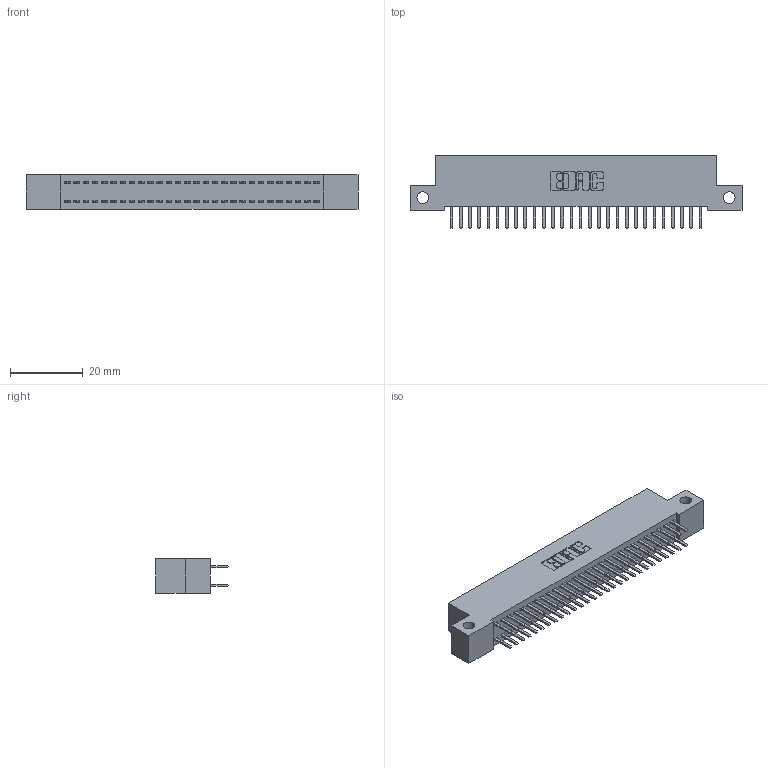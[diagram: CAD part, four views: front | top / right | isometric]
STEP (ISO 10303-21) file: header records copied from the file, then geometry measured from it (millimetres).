
FILE_DESCRIPTION (( 'STEP AP203' ), '1' );
FILE_NAME ('392-056-520-212.STEP', '2019-10-08T14:47:47', ( '' ), ( '' ), 'SwSTEP 2.0', 'SolidWorks 2016', '' );
FILE_SCHEMA (( 'CONFIG_CONTROL_DESIGN' ));
Length unit declared in the file: inch
Products named in the file (3): 342 Part_Side Mount; 345-292-001_345-293-120; 392-056-520-212
Assembly tree (57 placements, depth 2):
  392-056-520-212
    342 Part_Side Mount
    345-292-001_345-293-120  x56
Bounding box: 91.44 x 20.02 x 9.4 mm (x, y, z)
Volume: 8051.1 mm3; surface area: 12542.3 mm2
Topology: 57 solids, 57 shells, 3246 faces, 9427 edges, 6134 vertices
Faces by surface type: plane 2194, cylinder 1052
Entity records: 19809 total; most frequent: CARTESIAN_POINT 3310, ORIENTED_EDGE 3234, DIRECTION 2841, EDGE_CURVE 1617, VECTOR 1485, LINE 1485, VERTEX_POINT 1074, AXIS2_PLACEMENT_3D 678
